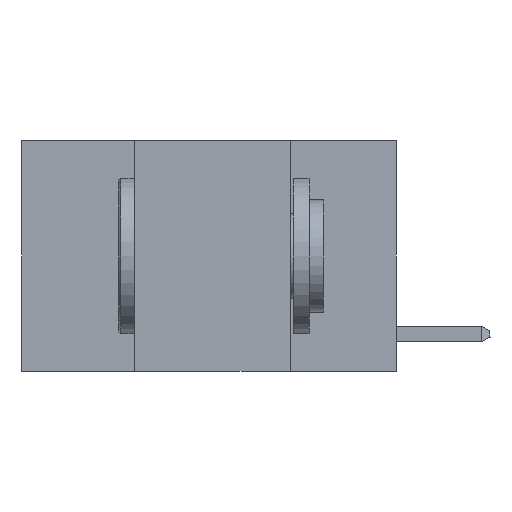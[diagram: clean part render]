
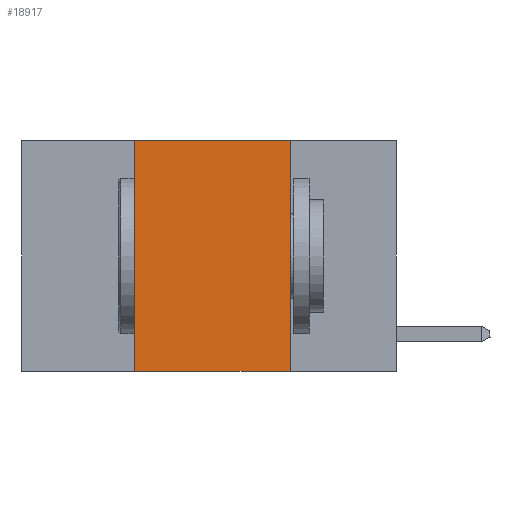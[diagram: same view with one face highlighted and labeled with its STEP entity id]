
A CAD part, left-side view. The second image highlights one B-rep face of the part: STEP entity #18917.
In plain terms, the highlighted planar face has unit normal (-1, 0, 0).
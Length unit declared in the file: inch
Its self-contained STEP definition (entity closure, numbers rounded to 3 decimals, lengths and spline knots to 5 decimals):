
#1145 = DIRECTION ( 'NONE',  ( 0., -1., 0. ) ) ;
#1175 = DIRECTION ( 'NONE',  ( 0., 0., -1. ) ) ;
#1247 = LINE ( 'NONE', #10788, #4160 ) ;
#2073 = PLANE ( 'NONE',  #19515 ) ;
#2208 = EDGE_CURVE ( 'NONE', #13027, #16333, #5382, .T. ) ;
#2495 = VECTOR ( 'NONE', #8633, 39.37008 ) ;
#3270 = EDGE_CURVE ( 'NONE', #15052, #6575, #4316, .T. ) ;
#4094 = ORIENTED_EDGE ( 'NONE', *, *, #3270, .F. ) ;
#4160 = VECTOR ( 'NONE', #21115, 39.37008 ) ;
#4316 = LINE ( 'NONE', #9308, #12920 ) ;
#5382 = LINE ( 'NONE', #15136, #2495 ) ;
#6022 = EDGE_CURVE ( 'NONE', #16333, #15052, #1247, .T. ) ;
#6248 = CARTESIAN_POINT ( 'NONE',  ( 0., 0.6, -0.37 ) ) ;
#6575 = VERTEX_POINT ( 'NONE', #14218 ) ;
#8633 = DIRECTION ( 'NONE',  ( 0., 0., 1. ) ) ;
#8692 = ORIENTED_EDGE ( 'NONE', *, *, #2208, .F. ) ;
#9168 = LINE ( 'NONE', #6248, #12444 ) ;
#9308 = CARTESIAN_POINT ( 'NONE',  ( 0., 0.17, 0. ) ) ;
#10524 = EDGE_LOOP ( 'NONE', ( #4094, #15651, #8692, #13309 ) ) ;
#10788 = CARTESIAN_POINT ( 'NONE',  ( 0., 0.6, 0. ) ) ;
#11197 = CARTESIAN_POINT ( 'NONE',  ( 0., 0.17, 0. ) ) ;
#12444 = VECTOR ( 'NONE', #1145, 39.37008 ) ;
#12920 = VECTOR ( 'NONE', #1175, 39.37008 ) ;
#13027 = VERTEX_POINT ( 'NONE', #13999 ) ;
#13309 = ORIENTED_EDGE ( 'NONE', *, *, #17682, .T. ) ;
#13665 = CARTESIAN_POINT ( 'NONE',  ( 0., 0.6, 0. ) ) ;
#13999 = CARTESIAN_POINT ( 'NONE',  ( 0., 0.42, -0.37 ) ) ;
#14218 = CARTESIAN_POINT ( 'NONE',  ( 0., 0.17, -0.37 ) ) ;
#15052 = VERTEX_POINT ( 'NONE', #11197 ) ;
#15136 = CARTESIAN_POINT ( 'NONE',  ( 0., 0.42, 0. ) ) ;
#15198 = FACE_OUTER_BOUND ( 'NONE', #10524, .T. ) ;
#15651 = ORIENTED_EDGE ( 'NONE', *, *, #6022, .F. ) ;
#16333 = VERTEX_POINT ( 'NONE', #18404 ) ;
#16630 = DIRECTION ( 'NONE',  ( 1., 0., 0. ) ) ;
#16835 = DIRECTION ( 'NONE',  ( 0., 0., -1. ) ) ;
#17682 = EDGE_CURVE ( 'NONE', #13027, #6575, #9168, .T. ) ;
#18404 = CARTESIAN_POINT ( 'NONE',  ( 0., 0.42, 0. ) ) ;
#18917 = ADVANCED_FACE ( 'NONE', ( #15198 ), #2073, .F. ) ;
#19515 = AXIS2_PLACEMENT_3D ( 'NONE', #13665, #16630, #16835 ) ;
#21115 = DIRECTION ( 'NONE',  ( 0., -1., 0. ) ) ;
